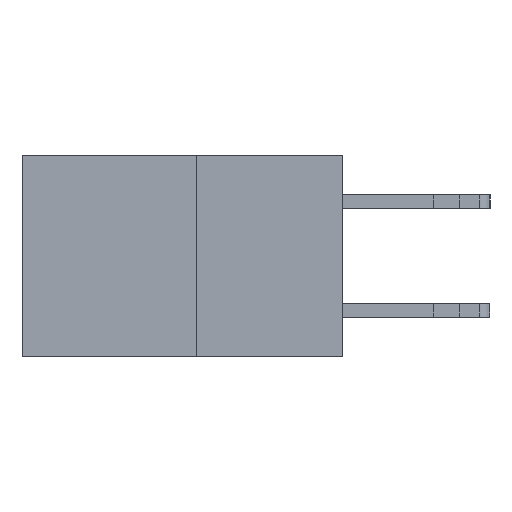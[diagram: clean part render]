
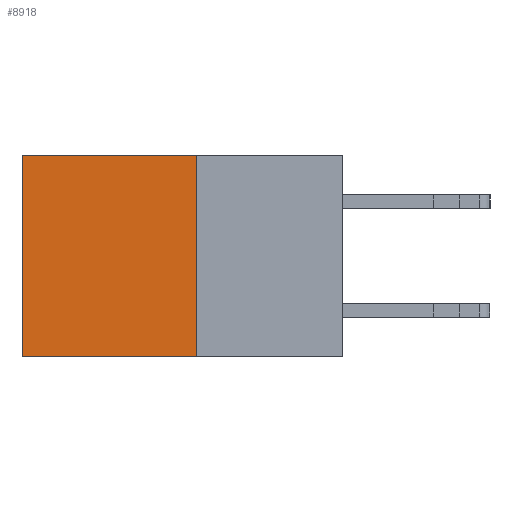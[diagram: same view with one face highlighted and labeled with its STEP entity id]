
A CAD part, left-side view. The second image highlights one B-rep face of the part: STEP entity #8918.
In plain terms, the highlighted planar face has unit normal (-1, 0, 0).
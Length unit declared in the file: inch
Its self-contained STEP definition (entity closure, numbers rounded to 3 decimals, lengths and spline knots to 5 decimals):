
#812 = CARTESIAN_POINT ( 'NONE',  ( 0.277, 0.27, -0.37 ) ) ;
#1074 = CARTESIAN_POINT ( 'NONE',  ( 0.277, 0.27, 0. ) ) ;
#1209 = AXIS2_PLACEMENT_3D ( 'NONE', #11326, #3144, #12644 ) ;
#1219 = VECTOR ( 'NONE', #17350, 39.37008 ) ;
#1779 = PLANE ( 'NONE',  #1209 ) ;
#1921 = VECTOR ( 'NONE', #8739, 39.37008 ) ;
#2010 = VERTEX_POINT ( 'NONE', #12113 ) ;
#2298 = EDGE_CURVE ( 'NONE', #10638, #14346, #6034, .T. ) ;
#3144 = DIRECTION ( 'NONE',  ( 1., 0., 0. ) ) ;
#3875 = CARTESIAN_POINT ( 'NONE',  ( 0.277, 0.27, -0.37 ) ) ;
#4936 = VECTOR ( 'NONE', #6675, 39.37008 ) ;
#5280 = CARTESIAN_POINT ( 'NONE',  ( 0.277, 0.27, 0. ) ) ;
#5339 = EDGE_LOOP ( 'NONE', ( #11059, #9951, #16636, #10750 ) ) ;
#5370 = LINE ( 'NONE', #5280, #4936 ) ;
#5662 = DIRECTION ( 'NONE',  ( 0., 0., -1. ) ) ;
#6034 = LINE ( 'NONE', #10294, #1921 ) ;
#6130 = CARTESIAN_POINT ( 'NONE',  ( 0.277, 0.59, 0. ) ) ;
#6675 = DIRECTION ( 'NONE',  ( 0., 1., 0. ) ) ;
#8597 = LINE ( 'NONE', #3875, #1219 ) ;
#8610 = VECTOR ( 'NONE', #5662, 39.37008 ) ;
#8739 = DIRECTION ( 'NONE',  ( 0., 0., -1. ) ) ;
#8918 = ADVANCED_FACE ( 'NONE', ( #14879 ), #1779, .F. ) ;
#9289 = EDGE_CURVE ( 'NONE', #10638, #16152, #5370, .T. ) ;
#9324 = EDGE_CURVE ( 'NONE', #14346, #2010, #8597, .T. ) ;
#9951 = ORIENTED_EDGE ( 'NONE', *, *, #9324, .F. ) ;
#10294 = CARTESIAN_POINT ( 'NONE',  ( 0.277, 0.27, -0.37 ) ) ;
#10638 = VERTEX_POINT ( 'NONE', #1074 ) ;
#10750 = ORIENTED_EDGE ( 'NONE', *, *, #9289, .T. ) ;
#11059 = ORIENTED_EDGE ( 'NONE', *, *, #13352, .T. ) ;
#11060 = CARTESIAN_POINT ( 'NONE',  ( 0.277, 0.59, -0.37 ) ) ;
#11326 = CARTESIAN_POINT ( 'NONE',  ( 0.277, 0.27, -0.37 ) ) ;
#12113 = CARTESIAN_POINT ( 'NONE',  ( 0.277, 0.59, -0.37 ) ) ;
#12644 = DIRECTION ( 'NONE',  ( 0., 0., -1. ) ) ;
#13352 = EDGE_CURVE ( 'NONE', #16152, #2010, #15705, .T. ) ;
#14346 = VERTEX_POINT ( 'NONE', #812 ) ;
#14879 = FACE_OUTER_BOUND ( 'NONE', #5339, .T. ) ;
#15705 = LINE ( 'NONE', #11060, #8610 ) ;
#16152 = VERTEX_POINT ( 'NONE', #6130 ) ;
#16636 = ORIENTED_EDGE ( 'NONE', *, *, #2298, .F. ) ;
#17350 = DIRECTION ( 'NONE',  ( 0., 1., 0. ) ) ;
